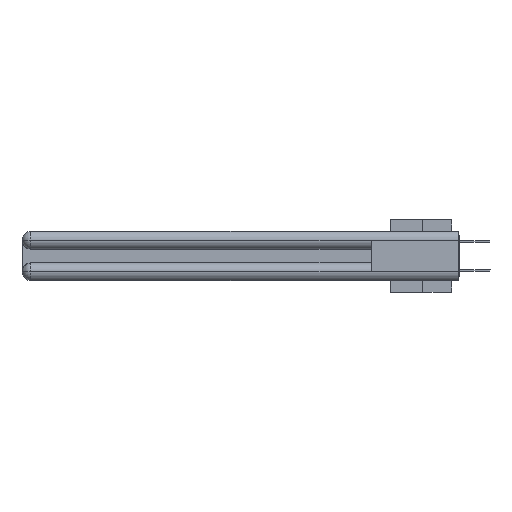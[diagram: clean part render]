
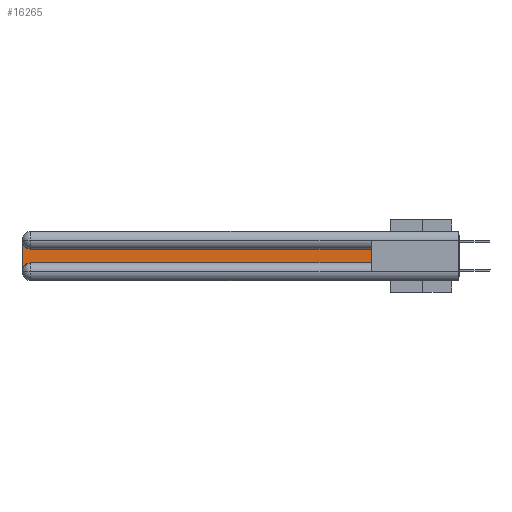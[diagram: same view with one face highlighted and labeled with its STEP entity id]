
A CAD part, left-side view. The second image highlights one B-rep face of the part: STEP entity #16265.
In plain terms, the highlighted planar face has unit normal (-1, 0, 0).
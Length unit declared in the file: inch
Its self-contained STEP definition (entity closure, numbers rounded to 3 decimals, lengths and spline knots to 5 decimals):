
#1115 = ORIENTED_EDGE ( 'NONE', *, *, #14170, .T. ) ;
#1303 = LINE ( 'NONE', #12313, #21631 ) ;
#1694 = DIRECTION ( 'NONE',  ( 0., 0., -1. ) ) ;
#2102 = EDGE_LOOP ( 'NONE', ( #34538, #1115, #15759, #27120, #11181, #3552 ) ) ;
#2132 = DIRECTION ( 'NONE',  ( 0., 0., -1. ) ) ;
#2275 = CARTESIAN_POINT ( 'NONE',  ( 0.075, 2.94, -0.0625 ) ) ;
#2504 = VERTEX_POINT ( 'NONE', #19756 ) ;
#2904 = VERTEX_POINT ( 'NONE', #5382 ) ;
#3277 = CARTESIAN_POINT ( 'NONE',  ( 0.075, 2.94, -0.1225 ) ) ;
#3552 = ORIENTED_EDGE ( 'NONE', *, *, #7652, .T. ) ;
#5187 = LINE ( 'NONE', #39377, #26056 ) ;
#5382 = CARTESIAN_POINT ( 'NONE',  ( 0.075, 3., -0.0625 ) ) ;
#5496 = LINE ( 'NONE', #39075, #28843 ) ;
#5786 = EDGE_CURVE ( 'NONE', #30348, #21586, #1303, .T. ) ;
#7652 = EDGE_CURVE ( 'NONE', #21586, #2504, #5187, .T. ) ;
#8414 = DIRECTION ( 'NONE',  ( 0., 0., 1. ) ) ;
#8602 = EDGE_CURVE ( 'NONE', #2904, #34142, #5496, .T. ) ;
#10732 = EDGE_CURVE ( 'NONE', #2504, #39198, #30446, .T. ) ;
#11181 = ORIENTED_EDGE ( 'NONE', *, *, #5786, .T. ) ;
#11433 = FACE_OUTER_BOUND ( 'NONE', #2102, .T. ) ;
#12212 = DIRECTION ( 'NONE',  ( 0., 1., 0. ) ) ;
#12313 = CARTESIAN_POINT ( 'NONE',  ( 0.075, 0.6, -0.2175 ) ) ;
#14170 = EDGE_CURVE ( 'NONE', #39198, #2904, #15903, .T. ) ;
#15759 = ORIENTED_EDGE ( 'NONE', *, *, #8602, .T. ) ;
#15903 = CIRCLE ( 'NONE', #29491, 0.06 ) ;
#16175 = VECTOR ( 'NONE', #12212, 39.37008 ) ;
#16265 = ADVANCED_FACE ( 'NONE', ( #11433 ), #35920, .F. ) ;
#17510 = CARTESIAN_POINT ( 'NONE',  ( 0.075, 3., -0.1225 ) ) ;
#18190 = DIRECTION ( 'NONE',  ( 1., 0., 0. ) ) ;
#19756 = CARTESIAN_POINT ( 'NONE',  ( 0.075, 0.6, -0.1225 ) ) ;
#21213 = CARTESIAN_POINT ( 'NONE',  ( 0.075, 2.94, -0.2775 ) ) ;
#21586 = VERTEX_POINT ( 'NONE', #26123 ) ;
#21631 = VECTOR ( 'NONE', #22210, 39.37008 ) ;
#22210 = DIRECTION ( 'NONE',  ( 0., -1., 0. ) ) ;
#23012 = CARTESIAN_POINT ( 'NONE',  ( 0.075, 2.94, -0.2175 ) ) ;
#23683 = DIRECTION ( 'NONE',  ( 0., 0., -1. ) ) ;
#26056 = VECTOR ( 'NONE', #8414, 39.37008 ) ;
#26123 = CARTESIAN_POINT ( 'NONE',  ( 0.075, 0.6, -0.2175 ) ) ;
#27120 = ORIENTED_EDGE ( 'NONE', *, *, #38293, .T. ) ;
#28843 = VECTOR ( 'NONE', #23683, 39.37008 ) ;
#29491 = AXIS2_PLACEMENT_3D ( 'NONE', #2275, #39105, #1694 ) ;
#29854 = DIRECTION ( 'NONE',  ( 1., 0., 0. ) ) ;
#30348 = VERTEX_POINT ( 'NONE', #23012 ) ;
#30446 = LINE ( 'NONE', #33453, #16175 ) ;
#32599 = CIRCLE ( 'NONE', #35833, 0.06 ) ;
#33453 = CARTESIAN_POINT ( 'NONE',  ( 0.075, 0.6, -0.1225 ) ) ;
#33758 = DIRECTION ( 'NONE',  ( 0., 0., -1. ) ) ;
#34142 = VERTEX_POINT ( 'NONE', #39831 ) ;
#34538 = ORIENTED_EDGE ( 'NONE', *, *, #10732, .T. ) ;
#34792 = AXIS2_PLACEMENT_3D ( 'NONE', #17510, #29854, #2132 ) ;
#35833 = AXIS2_PLACEMENT_3D ( 'NONE', #21213, #18190, #33758 ) ;
#35920 = PLANE ( 'NONE',  #34792 ) ;
#38293 = EDGE_CURVE ( 'NONE', #34142, #30348, #32599, .T. ) ;
#39075 = CARTESIAN_POINT ( 'NONE',  ( 0.075, 3., -0.2175 ) ) ;
#39105 = DIRECTION ( 'NONE',  ( 1., 0., 0. ) ) ;
#39198 = VERTEX_POINT ( 'NONE', #3277 ) ;
#39377 = CARTESIAN_POINT ( 'NONE',  ( 0.075, 0.6, -0.2175 ) ) ;
#39831 = CARTESIAN_POINT ( 'NONE',  ( 0.075, 3., -0.2775 ) ) ;
